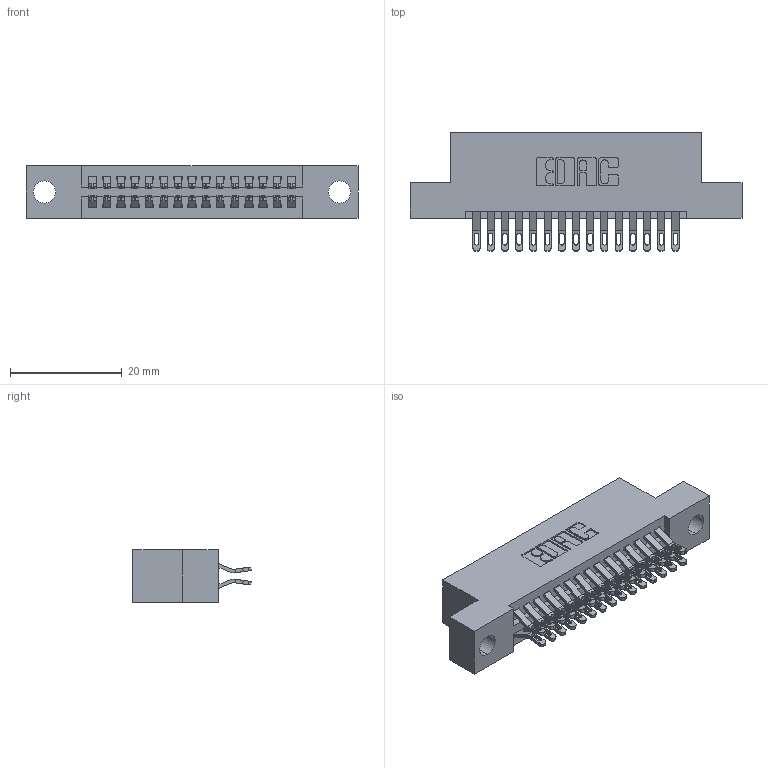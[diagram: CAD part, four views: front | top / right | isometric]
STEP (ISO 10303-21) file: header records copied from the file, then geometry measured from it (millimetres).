
FILE_DESCRIPTION (( 'STEP AP203' ), '1' );
FILE_NAME ('395-030-555-204.STEP', '2018-11-11T07:03:38', ( '' ), ( '' ), 'SwSTEP 2.0', 'SolidWorks 2016', '' );
FILE_SCHEMA (( 'CONFIG_CONTROL_DESIGN' ));
Length unit declared in the file: inch
Products named in the file (3): 345-292-001_555 Tail; 395-030-555-204; 345 Part_Flush Mounting Lugs - 0.156 Dia-TH
Assembly tree (31 placements, depth 2):
  395-030-555-204
    345 Part_Flush Mounting Lugs - 0.156 Dia-TH
    345-292-001_555 Tail  x30
Bounding box: 59.31 x 21.13 x 9.4 mm (x, y, z)
Volume: 5509.9 mm3; surface area: 7739.4 mm2
Topology: 31 solids, 31 shells, 1806 faces, 5651 edges, 3766 vertices
Faces by surface type: plane 1010, cylinder 796
Entity records: 15733 total; most frequent: CARTESIAN_POINT 2698, ORIENTED_EDGE 2602, DIRECTION 2381, EDGE_CURVE 1301, VECTOR 1089, LINE 1089, VERTEX_POINT 866, AXIS2_PLACEMENT_3D 646
